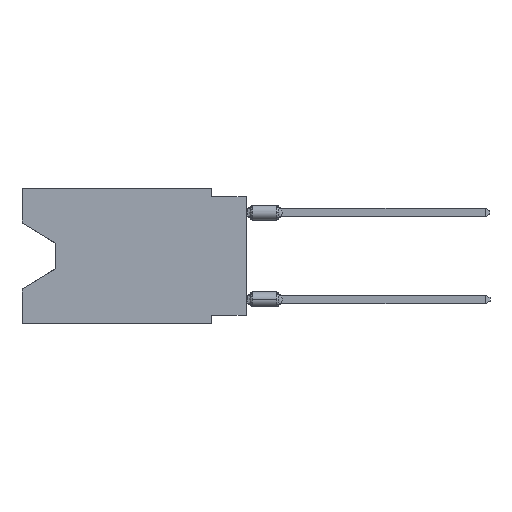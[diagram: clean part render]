
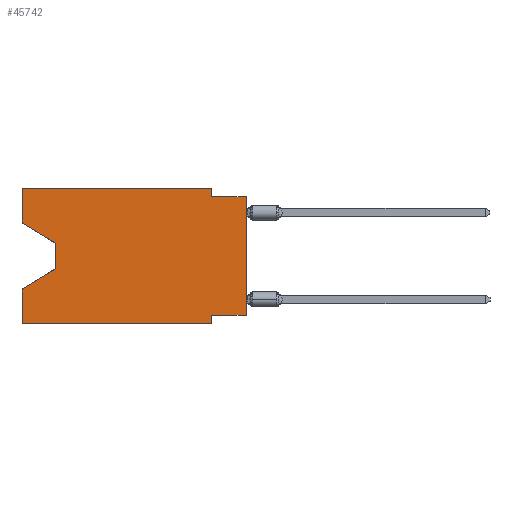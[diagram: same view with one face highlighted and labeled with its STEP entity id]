
A CAD part, left-side view. The second image highlights one B-rep face of the part: STEP entity #45742.
In plain terms, the highlighted planar face has unit normal (-1, 0, 0).
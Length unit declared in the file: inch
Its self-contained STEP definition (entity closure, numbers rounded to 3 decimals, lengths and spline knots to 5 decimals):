
#137 = ORIENTED_EDGE ( 'NONE', *, *, #38176, .F. ) ;
#1066 = ORIENTED_EDGE ( 'NONE', *, *, #57275, .T. ) ;
#1964 = VECTOR ( 'NONE', #39592, 39.37008 ) ;
#2085 = DIRECTION ( 'NONE',  ( 0., -1., 0. ) ) ;
#2420 = LINE ( 'NONE', #23975, #6982 ) ;
#2596 = DIRECTION ( 'NONE',  ( 0., 0., -1. ) ) ;
#3193 = LINE ( 'NONE', #8337, #15205 ) ;
#4068 = ORIENTED_EDGE ( 'NONE', *, *, #25247, .F. ) ;
#4144 = EDGE_CURVE ( 'NONE', #17363, #39774, #16947, .T. ) ;
#5415 = LINE ( 'NONE', #47163, #17083 ) ;
#6429 = EDGE_CURVE ( 'NONE', #9162, #58130, #66351, .T. ) ;
#6653 = CARTESIAN_POINT ( 'NONE',  ( 0., 0.645, 0. ) ) ;
#6982 = VECTOR ( 'NONE', #7894, 39.37008 ) ;
#6990 = CARTESIAN_POINT ( 'NONE',  ( 0., 0.1, 0. ) ) ;
#7894 = DIRECTION ( 'NONE',  ( 0., 0., -1. ) ) ;
#8337 = CARTESIAN_POINT ( 'NONE',  ( 0., 0.645, 0. ) ) ;
#8785 = ORIENTED_EDGE ( 'NONE', *, *, #6429, .T. ) ;
#9162 = VERTEX_POINT ( 'NONE', #47248 ) ;
#9629 = CARTESIAN_POINT ( 'NONE',  ( 0., 0.645, 0. ) ) ;
#9868 = CARTESIAN_POINT ( 'NONE',  ( 0., 0.55, -0.232 ) ) ;
#9968 = CARTESIAN_POINT ( 'NONE',  ( 0., 0.55, -0.158 ) ) ;
#10061 = VERTEX_POINT ( 'NONE', #21779 ) ;
#12536 = CARTESIAN_POINT ( 'NONE',  ( 0., 0.1, 0. ) ) ;
#12816 = DIRECTION ( 'NONE',  ( 0., 0., 1. ) ) ;
#12941 = EDGE_CURVE ( 'NONE', #57184, #39774, #20422, .T. ) ;
#12981 = CARTESIAN_POINT ( 'NONE',  ( 0., 0.645, -0.10025 ) ) ;
#15205 = VECTOR ( 'NONE', #12816, 39.37008 ) ;
#15499 = DIRECTION ( 'NONE',  ( 0., -1., 0. ) ) ;
#15999 = DIRECTION ( 'NONE',  ( 0., 1., 0. ) ) ;
#16947 = LINE ( 'NONE', #6653, #37001 ) ;
#17083 = VECTOR ( 'NONE', #21155, 39.37008 ) ;
#17363 = VERTEX_POINT ( 'NONE', #33760 ) ;
#18267 = VERTEX_POINT ( 'NONE', #50354 ) ;
#18875 = FACE_OUTER_BOUND ( 'NONE', #48834, .T. ) ;
#19395 = LINE ( 'NONE', #44737, #1964 ) ;
#19942 = LINE ( 'NONE', #62052, #65643 ) ;
#20422 = LINE ( 'NONE', #61832, #47901 ) ;
#20774 = ORIENTED_EDGE ( 'NONE', *, *, #66841, .T. ) ;
#21155 = DIRECTION ( 'NONE',  ( 0., 0., -1. ) ) ;
#21779 = CARTESIAN_POINT ( 'NONE',  ( 0., 0., -0.025 ) ) ;
#22934 = CARTESIAN_POINT ( 'NONE',  ( 0., 0.1, -0.365 ) ) ;
#23975 = CARTESIAN_POINT ( 'NONE',  ( 0., 0.1, -0.39 ) ) ;
#24903 = CARTESIAN_POINT ( 'NONE',  ( 0., 0., -0.365 ) ) ;
#25247 = EDGE_CURVE ( 'NONE', #25289, #51050, #62880, .T. ) ;
#25289 = VERTEX_POINT ( 'NONE', #24903 ) ;
#29936 = VECTOR ( 'NONE', #2085, 39.37008 ) ;
#32453 = VERTEX_POINT ( 'NONE', #6990 ) ;
#32680 = LINE ( 'NONE', #34084, #61068 ) ;
#32927 = ORIENTED_EDGE ( 'NONE', *, *, #61151, .F. ) ;
#33760 = CARTESIAN_POINT ( 'NONE',  ( 0., 0.645, -0.39 ) ) ;
#33896 = LINE ( 'NONE', #54789, #29936 ) ;
#34084 = CARTESIAN_POINT ( 'NONE',  ( 0., 0., 0. ) ) ;
#34182 = DIRECTION ( 'NONE',  ( 0., -0.855, -0.519 ) ) ;
#35275 = DIRECTION ( 'NONE',  ( 1., 0., 0. ) ) ;
#35423 = DIRECTION ( 'NONE',  ( 0., 0., 1. ) ) ;
#37001 = VECTOR ( 'NONE', #59018, 39.37008 ) ;
#38110 = EDGE_CURVE ( 'NONE', #51050, #59030, #2420, .T. ) ;
#38176 = EDGE_CURVE ( 'NONE', #61009, #10061, #33896, .T. ) ;
#38196 = LINE ( 'NONE', #12536, #61905 ) ;
#39592 = DIRECTION ( 'NONE',  ( 0., -1., 0. ) ) ;
#39774 = VERTEX_POINT ( 'NONE', #47540 ) ;
#40381 = EDGE_CURVE ( 'NONE', #32453, #61009, #38196, .T. ) ;
#43114 = VECTOR ( 'NONE', #15999, 39.37008 ) ;
#43406 = CARTESIAN_POINT ( 'NONE',  ( 0., 0.1, -0.025 ) ) ;
#44737 = CARTESIAN_POINT ( 'NONE',  ( 0., 0.645, 0. ) ) ;
#45586 = ORIENTED_EDGE ( 'NONE', *, *, #12941, .T. ) ;
#45742 = ADVANCED_FACE ( 'NONE', ( #18875 ), #60634, .F. ) ;
#45815 = AXIS2_PLACEMENT_3D ( 'NONE', #9629, #35275, #46245 ) ;
#46245 = DIRECTION ( 'NONE',  ( 0., 0., -1. ) ) ;
#47163 = CARTESIAN_POINT ( 'NONE',  ( 0., 0.55, -0.158 ) ) ;
#47248 = CARTESIAN_POINT ( 'NONE',  ( 0., 0.645, -0.10025 ) ) ;
#47540 = CARTESIAN_POINT ( 'NONE',  ( 0., 0.645, -0.28975 ) ) ;
#47901 = VECTOR ( 'NONE', #51915, 39.37008 ) ;
#48834 = EDGE_LOOP ( 'NONE', ( #8785, #1066, #45586, #64389, #20774, #52125, #4068, #57112, #137, #53818, #32927, #52116 ) ) ;
#49594 = VECTOR ( 'NONE', #34182, 39.37008 ) ;
#50354 = CARTESIAN_POINT ( 'NONE',  ( 0., 0.645, 0. ) ) ;
#51050 = VERTEX_POINT ( 'NONE', #22934 ) ;
#51915 = DIRECTION ( 'NONE',  ( 0., 0.855, -0.519 ) ) ;
#52116 = ORIENTED_EDGE ( 'NONE', *, *, #63123, .F. ) ;
#52125 = ORIENTED_EDGE ( 'NONE', *, *, #38110, .F. ) ;
#53818 = ORIENTED_EDGE ( 'NONE', *, *, #40381, .F. ) ;
#54789 = CARTESIAN_POINT ( 'NONE',  ( 0., 0., -0.025 ) ) ;
#57112 = ORIENTED_EDGE ( 'NONE', *, *, #62611, .T. ) ;
#57184 = VERTEX_POINT ( 'NONE', #9868 ) ;
#57275 = EDGE_CURVE ( 'NONE', #58130, #57184, #5415, .T. ) ;
#58130 = VERTEX_POINT ( 'NONE', #9968 ) ;
#59018 = DIRECTION ( 'NONE',  ( 0., 0., 1. ) ) ;
#59030 = VERTEX_POINT ( 'NONE', #66084 ) ;
#60634 = PLANE ( 'NONE',  #45815 ) ;
#61009 = VERTEX_POINT ( 'NONE', #43406 ) ;
#61068 = VECTOR ( 'NONE', #35423, 39.37008 ) ;
#61151 = EDGE_CURVE ( 'NONE', #18267, #32453, #19395, .T. ) ;
#61832 = CARTESIAN_POINT ( 'NONE',  ( 0., 0.55, -0.232 ) ) ;
#61856 = CARTESIAN_POINT ( 'NONE',  ( 0., 0., -0.365 ) ) ;
#61905 = VECTOR ( 'NONE', #2596, 39.37008 ) ;
#62052 = CARTESIAN_POINT ( 'NONE',  ( 0., 0.645, -0.39 ) ) ;
#62611 = EDGE_CURVE ( 'NONE', #25289, #10061, #32680, .T. ) ;
#62880 = LINE ( 'NONE', #61856, #43114 ) ;
#63123 = EDGE_CURVE ( 'NONE', #9162, #18267, #3193, .T. ) ;
#64389 = ORIENTED_EDGE ( 'NONE', *, *, #4144, .F. ) ;
#65643 = VECTOR ( 'NONE', #15499, 39.37008 ) ;
#66084 = CARTESIAN_POINT ( 'NONE',  ( 0., 0.1, -0.39 ) ) ;
#66351 = LINE ( 'NONE', #12981, #49594 ) ;
#66841 = EDGE_CURVE ( 'NONE', #17363, #59030, #19942, .T. ) ;
